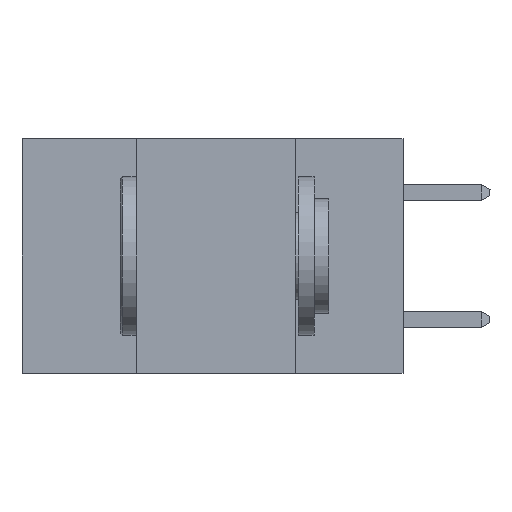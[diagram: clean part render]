
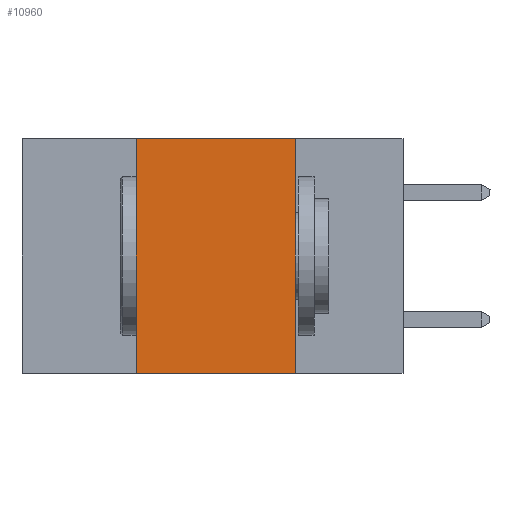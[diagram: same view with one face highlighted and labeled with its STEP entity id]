
A CAD part, left-side view. The second image highlights one B-rep face of the part: STEP entity #10960.
In plain terms, the highlighted planar face has unit normal (-1, 0, 0).
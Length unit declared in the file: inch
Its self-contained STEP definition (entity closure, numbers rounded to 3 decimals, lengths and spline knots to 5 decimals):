
#59 = EDGE_CURVE ( 'NONE', #19422, #4654, #9625, .T. ) ;
#589 = CARTESIAN_POINT ( 'NONE',  ( 0., 0.42, -0.37 ) ) ;
#990 = CARTESIAN_POINT ( 'NONE',  ( 0., 0.42, 0. ) ) ;
#3159 = CARTESIAN_POINT ( 'NONE',  ( 0., 0.17, -0.37 ) ) ;
#3395 = DIRECTION ( 'NONE',  ( 0., -1., 0. ) ) ;
#3906 = ORIENTED_EDGE ( 'NONE', *, *, #35709, .F. ) ;
#4654 = VERTEX_POINT ( 'NONE', #990 ) ;
#4817 = CARTESIAN_POINT ( 'NONE',  ( 0., 0.17, 0. ) ) ;
#6339 = VECTOR ( 'NONE', #3395, 39.37008 ) ;
#7517 = AXIS2_PLACEMENT_3D ( 'NONE', #22686, #19409, #38885 ) ;
#8895 = LINE ( 'NONE', #39299, #30510 ) ;
#8983 = VECTOR ( 'NONE', #33601, 39.37008 ) ;
#9625 = LINE ( 'NONE', #32743, #23035 ) ;
#10960 = ADVANCED_FACE ( 'NONE', ( #14533 ), #35540, .F. ) ;
#14533 = FACE_OUTER_BOUND ( 'NONE', #24243, .T. ) ;
#15163 = LINE ( 'NONE', #33395, #6339 ) ;
#16130 = ORIENTED_EDGE ( 'NONE', *, *, #59, .F. ) ;
#17343 = CARTESIAN_POINT ( 'NONE',  ( 0., 0.17, 0. ) ) ;
#18486 = VERTEX_POINT ( 'NONE', #3159 ) ;
#19260 = DIRECTION ( 'NONE',  ( 0., 0., 1. ) ) ;
#19409 = DIRECTION ( 'NONE',  ( 1., 0., 0. ) ) ;
#19422 = VERTEX_POINT ( 'NONE', #589 ) ;
#22183 = ORIENTED_EDGE ( 'NONE', *, *, #29271, .T. ) ;
#22686 = CARTESIAN_POINT ( 'NONE',  ( 0., 0.6, 0. ) ) ;
#22944 = DIRECTION ( 'NONE',  ( 0., -1., 0. ) ) ;
#23035 = VECTOR ( 'NONE', #19260, 39.37008 ) ;
#23130 = VERTEX_POINT ( 'NONE', #4817 ) ;
#24243 = EDGE_LOOP ( 'NONE', ( #33607, #3906, #16130, #22183 ) ) ;
#29271 = EDGE_CURVE ( 'NONE', #19422, #18486, #8895, .T. ) ;
#30510 = VECTOR ( 'NONE', #22944, 39.37008 ) ;
#32743 = CARTESIAN_POINT ( 'NONE',  ( 0., 0.42, 0. ) ) ;
#33395 = CARTESIAN_POINT ( 'NONE',  ( 0., 0.6, 0. ) ) ;
#33601 = DIRECTION ( 'NONE',  ( 0., 0., -1. ) ) ;
#33607 = ORIENTED_EDGE ( 'NONE', *, *, #33892, .F. ) ;
#33892 = EDGE_CURVE ( 'NONE', #23130, #18486, #36354, .T. ) ;
#35540 = PLANE ( 'NONE',  #7517 ) ;
#35709 = EDGE_CURVE ( 'NONE', #4654, #23130, #15163, .T. ) ;
#36354 = LINE ( 'NONE', #17343, #8983 ) ;
#38885 = DIRECTION ( 'NONE',  ( 0., 0., -1. ) ) ;
#39299 = CARTESIAN_POINT ( 'NONE',  ( 0., 0.6, -0.37 ) ) ;
